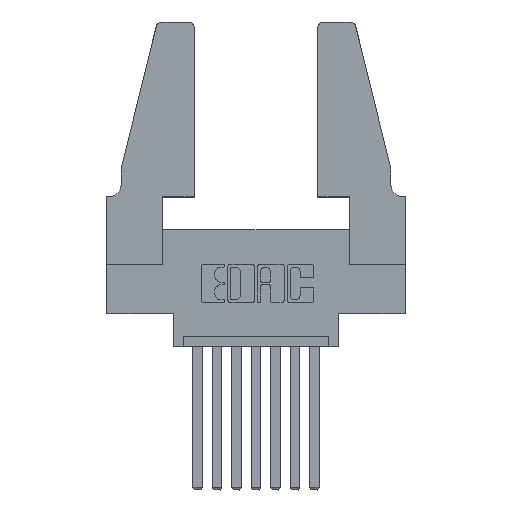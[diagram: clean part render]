
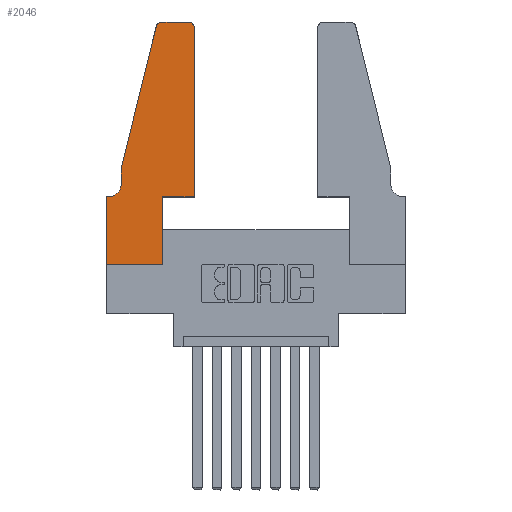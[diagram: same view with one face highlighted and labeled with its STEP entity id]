
A CAD part, top view. The second image highlights one B-rep face of the part: STEP entity #2046.
In plain terms, the highlighted planar face has unit normal (0, 0, 1).
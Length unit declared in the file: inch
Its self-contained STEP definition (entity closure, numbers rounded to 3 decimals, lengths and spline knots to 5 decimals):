
#31 = VERTEX_POINT ( 'NONE', #1451 ) ;
#32 = VERTEX_POINT ( 'NONE', #8025 ) ;
#137 = ORIENTED_EDGE ( 'NONE', *, *, #920, .T. ) ;
#185 = DIRECTION ( 'NONE',  ( -1., 0., 0. ) ) ;
#346 = CARTESIAN_POINT ( 'NONE',  ( 0.4505, 1.22, 0.37 ) ) ;
#773 = EDGE_CURVE ( 'NONE', #8553, #1974, #2251, .T. ) ;
#780 = CARTESIAN_POINT ( 'NONE',  ( 0.284, 1.22, 0.37 ) ) ;
#821 = CARTESIAN_POINT ( 'NONE',  ( 0.0755, 0.5, 0.37 ) ) ;
#824 = DIRECTION ( 'NONE',  ( 0., -1., 0. ) ) ;
#897 = VERTEX_POINT ( 'NONE', #11511 ) ;
#920 = EDGE_CURVE ( 'NONE', #11267, #1156, #9104, .T. ) ;
#1058 = ORIENTED_EDGE ( 'NONE', *, *, #5067, .T. ) ;
#1084 = FACE_OUTER_BOUND ( 'NONE', #9682, .T. ) ;
#1156 = VERTEX_POINT ( 'NONE', #6814 ) ;
#1294 = CARTESIAN_POINT ( 'NONE',  ( 0.4205, 1.22, 0.37 ) ) ;
#1338 = CARTESIAN_POINT ( 'NONE',  ( 0., 0.35, 0.37 ) ) ;
#1361 = LINE ( 'NONE', #5059, #6643 ) ;
#1451 = CARTESIAN_POINT ( 'NONE',  ( 0.2865, 0.35, 0.37 ) ) ;
#1546 = VERTEX_POINT ( 'NONE', #7523 ) ;
#1633 = AXIS2_PLACEMENT_3D ( 'NONE', #1294, #8766, #3126 ) ;
#1661 = LINE ( 'NONE', #2057, #11312 ) ;
#1865 = CARTESIAN_POINT ( 'NONE',  ( 0.0755, 0.42, 0.37 ) ) ;
#1954 = VERTEX_POINT ( 'NONE', #8167 ) ;
#1974 = VERTEX_POINT ( 'NONE', #10170 ) ;
#2007 = CARTESIAN_POINT ( 'NONE',  ( 0.2605, 1.25, 0.37 ) ) ;
#2046 = ADVANCED_FACE ( 'NONE', ( #1084 ), #9313, .T. ) ;
#2057 = CARTESIAN_POINT ( 'NONE',  ( 0.0755, 0.35, 0.37 ) ) ;
#2125 = EDGE_CURVE ( 'NONE', #1974, #6145, #1661, .T. ) ;
#2251 = CIRCLE ( 'NONE', #9216, 0.07 ) ;
#2353 = VECTOR ( 'NONE', #6456, 39.37008 ) ;
#2499 = ORIENTED_EDGE ( 'NONE', *, *, #5996, .T. ) ;
#2670 = EDGE_CURVE ( 'NONE', #31, #1954, #3565, .T. ) ;
#2826 = VECTOR ( 'NONE', #6594, 39.37008 ) ;
#2832 = AXIS2_PLACEMENT_3D ( 'NONE', #10257, #12064, #4815 ) ;
#2906 = ORIENTED_EDGE ( 'NONE', *, *, #2125, .T. ) ;
#3083 = VECTOR ( 'NONE', #824, 39.37008 ) ;
#3126 = DIRECTION ( 'NONE',  ( 1., 0., 0. ) ) ;
#3183 = AXIS2_PLACEMENT_3D ( 'NONE', #780, #6387, #11057 ) ;
#3191 = CARTESIAN_POINT ( 'NONE',  ( 0.25487, 1.22718, 0.37 ) ) ;
#3203 = ORIENTED_EDGE ( 'NONE', *, *, #2670, .T. ) ;
#3565 = LINE ( 'NONE', #7024, #6913 ) ;
#3937 = CARTESIAN_POINT ( 'NONE',  ( 0.0055, 0.42, 0.37 ) ) ;
#4407 = CARTESIAN_POINT ( 'NONE',  ( 0.0755, 0.5, 0.37 ) ) ;
#4815 = DIRECTION ( 'NONE',  ( 1., 0., 0. ) ) ;
#4846 = CARTESIAN_POINT ( 'NONE',  ( 0.0755, 0.5, 0.37 ) ) ;
#5029 = EDGE_CURVE ( 'NONE', #32, #11868, #11528, .T. ) ;
#5059 = CARTESIAN_POINT ( 'NONE',  ( 0.2865, 0.35, 0.37 ) ) ;
#5067 = EDGE_CURVE ( 'NONE', #6145, #1546, #10935, .T. ) ;
#5075 = ORIENTED_EDGE ( 'NONE', *, *, #9861, .T. ) ;
#5146 = DIRECTION ( 'NONE',  ( 0., 1., 0. ) ) ;
#5996 = EDGE_CURVE ( 'NONE', #1954, #11267, #7272, .T. ) ;
#6145 = VERTEX_POINT ( 'NONE', #1338 ) ;
#6163 = DIRECTION ( 'NONE',  ( 1., 0., 0. ) ) ;
#6387 = DIRECTION ( 'NONE',  ( 0., 0., 1. ) ) ;
#6456 = DIRECTION ( 'NONE',  ( 0., -1., 0. ) ) ;
#6594 = DIRECTION ( 'NONE',  ( -1., 0., 0. ) ) ;
#6643 = VECTOR ( 'NONE', #5146, 39.37008 ) ;
#6814 = CARTESIAN_POINT ( 'NONE',  ( 0.4205, 1.25, 0.37 ) ) ;
#6884 = LINE ( 'NONE', #821, #2353 ) ;
#6913 = VECTOR ( 'NONE', #6163, 39.37008 ) ;
#7024 = CARTESIAN_POINT ( 'NONE',  ( 0.4505, 0.35, 0.37 ) ) ;
#7272 = LINE ( 'NONE', #10981, #7711 ) ;
#7523 = CARTESIAN_POINT ( 'NONE',  ( 0., 0., 0.37 ) ) ;
#7711 = VECTOR ( 'NONE', #8041, 39.37008 ) ;
#8025 = CARTESIAN_POINT ( 'NONE',  ( 0.284, 1.25, 0.37 ) ) ;
#8026 = CARTESIAN_POINT ( 'NONE',  ( 0., 0., 0.37 ) ) ;
#8041 = DIRECTION ( 'NONE',  ( 0., 1., 0. ) ) ;
#8061 = LINE ( 'NONE', #8026, #10260 ) ;
#8167 = CARTESIAN_POINT ( 'NONE',  ( 0.4505, 0.35, 0.37 ) ) ;
#8553 = VERTEX_POINT ( 'NONE', #1865 ) ;
#8766 = DIRECTION ( 'NONE',  ( 0., 0., 1. ) ) ;
#8799 = DIRECTION ( 'NONE',  ( 1., 0., 0. ) ) ;
#9104 = CIRCLE ( 'NONE', #1633, 0.03 ) ;
#9125 = LINE ( 'NONE', #4407, #11469 ) ;
#9152 = EDGE_CURVE ( 'NONE', #11868, #9772, #9125, .T. ) ;
#9216 = AXIS2_PLACEMENT_3D ( 'NONE', #3937, #10461, #9520 ) ;
#9313 = PLANE ( 'NONE',  #2832 ) ;
#9520 = DIRECTION ( 'NONE',  ( -1., 0., 0. ) ) ;
#9673 = LINE ( 'NONE', #2007, #2826 ) ;
#9682 = EDGE_LOOP ( 'NONE', ( #11237, #11597, #10237, #11344, #10723, #2906, #1058, #10777, #5075, #3203, #2499, #137 ) ) ;
#9772 = VERTEX_POINT ( 'NONE', #4846 ) ;
#9861 = EDGE_CURVE ( 'NONE', #897, #31, #1361, .T. ) ;
#10170 = CARTESIAN_POINT ( 'NONE',  ( 0.0055, 0.35, 0.37 ) ) ;
#10199 = CARTESIAN_POINT ( 'NONE',  ( 0., 0., 0.37 ) ) ;
#10237 = ORIENTED_EDGE ( 'NONE', *, *, #9152, .T. ) ;
#10257 = CARTESIAN_POINT ( 'NONE',  ( 0., 0.35, 0.37 ) ) ;
#10260 = VECTOR ( 'NONE', #8799, 39.37008 ) ;
#10461 = DIRECTION ( 'NONE',  ( 0., 0., -1. ) ) ;
#10509 = EDGE_CURVE ( 'NONE', #1156, #32, #9673, .T. ) ;
#10679 = EDGE_CURVE ( 'NONE', #1546, #897, #8061, .T. ) ;
#10723 = ORIENTED_EDGE ( 'NONE', *, *, #773, .T. ) ;
#10777 = ORIENTED_EDGE ( 'NONE', *, *, #10679, .T. ) ;
#10871 = DIRECTION ( 'NONE',  ( -0.239, -0.971, 0. ) ) ;
#10935 = LINE ( 'NONE', #10199, #3083 ) ;
#10981 = CARTESIAN_POINT ( 'NONE',  ( 0.4505, 0.35, 0.37 ) ) ;
#11057 = DIRECTION ( 'NONE',  ( 1., 0., 0. ) ) ;
#11237 = ORIENTED_EDGE ( 'NONE', *, *, #10509, .T. ) ;
#11267 = VERTEX_POINT ( 'NONE', #346 ) ;
#11312 = VECTOR ( 'NONE', #185, 39.37008 ) ;
#11344 = ORIENTED_EDGE ( 'NONE', *, *, #11552, .T. ) ;
#11469 = VECTOR ( 'NONE', #10871, 39.37008 ) ;
#11511 = CARTESIAN_POINT ( 'NONE',  ( 0.2865, 0., 0.37 ) ) ;
#11528 = CIRCLE ( 'NONE', #3183, 0.03 ) ;
#11552 = EDGE_CURVE ( 'NONE', #9772, #8553, #6884, .T. ) ;
#11597 = ORIENTED_EDGE ( 'NONE', *, *, #5029, .T. ) ;
#11868 = VERTEX_POINT ( 'NONE', #3191 ) ;
#12064 = DIRECTION ( 'NONE',  ( 0., 0., 1. ) ) ;
